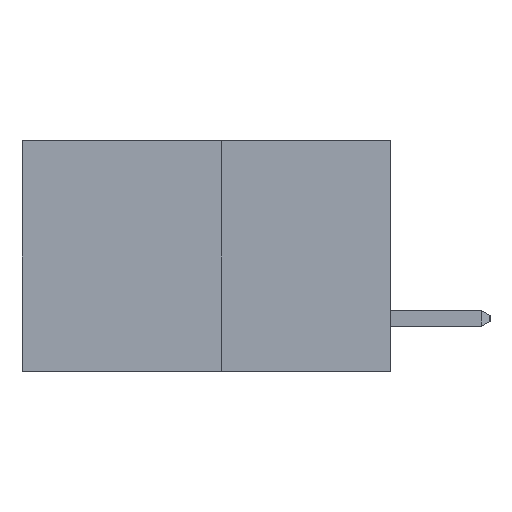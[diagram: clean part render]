
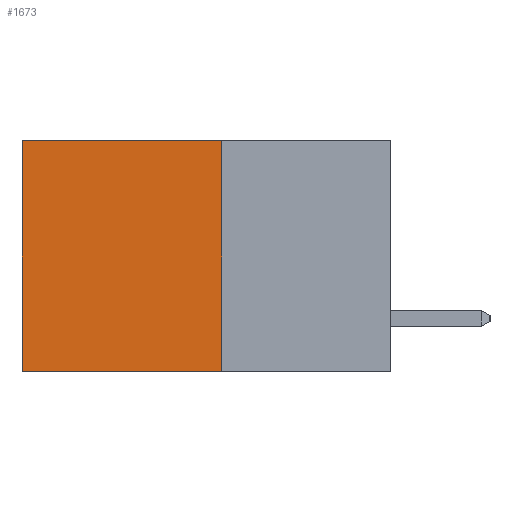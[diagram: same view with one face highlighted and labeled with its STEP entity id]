
A CAD part, left-side view. The second image highlights one B-rep face of the part: STEP entity #1673.
In plain terms, the highlighted planar face has unit normal (-1, 0, 0).
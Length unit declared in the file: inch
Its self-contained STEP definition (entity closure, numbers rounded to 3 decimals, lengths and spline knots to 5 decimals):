
#205 = LINE ( 'NONE', #525, #10479 ) ;
#525 = CARTESIAN_POINT ( 'NONE',  ( 0.277, 0.59, -0.37 ) ) ;
#1428 = VECTOR ( 'NONE', #2222, 39.37008 ) ;
#1673 = ADVANCED_FACE ( 'NONE', ( #11028 ), #9354, .F. ) ;
#1768 = VECTOR ( 'NONE', #6819, 39.37008 ) ;
#2113 = CARTESIAN_POINT ( 'NONE',  ( 0.277, 0.27, -0.37 ) ) ;
#2222 = DIRECTION ( 'NONE',  ( 0., 0., -1. ) ) ;
#2386 = LINE ( 'NONE', #12180, #1428 ) ;
#3002 = ORIENTED_EDGE ( 'NONE', *, *, #8285, .F. ) ;
#3289 = EDGE_CURVE ( 'NONE', #11826, #7920, #2386, .T. ) ;
#3498 = EDGE_CURVE ( 'NONE', #11826, #4639, #9947, .T. ) ;
#3953 = ORIENTED_EDGE ( 'NONE', *, *, #3498, .T. ) ;
#4101 = EDGE_LOOP ( 'NONE', ( #10529, #3002, #9128, #3953 ) ) ;
#4295 = AXIS2_PLACEMENT_3D ( 'NONE', #9626, #9228, #6537 ) ;
#4399 = CARTESIAN_POINT ( 'NONE',  ( 0.277, 0.27, -0.37 ) ) ;
#4639 = VERTEX_POINT ( 'NONE', #7911 ) ;
#5993 = VECTOR ( 'NONE', #12181, 39.37008 ) ;
#6537 = DIRECTION ( 'NONE',  ( 0., 0., -1. ) ) ;
#6768 = DIRECTION ( 'NONE',  ( 0., 0., -1. ) ) ;
#6819 = DIRECTION ( 'NONE',  ( 0., 1., 0. ) ) ;
#7879 = VERTEX_POINT ( 'NONE', #9518 ) ;
#7911 = CARTESIAN_POINT ( 'NONE',  ( 0.277, 0.59, 0. ) ) ;
#7920 = VERTEX_POINT ( 'NONE', #4399 ) ;
#8285 = EDGE_CURVE ( 'NONE', #7920, #7879, #8729, .T. ) ;
#8370 = CARTESIAN_POINT ( 'NONE',  ( 0.277, 0.27, 0. ) ) ;
#8729 = LINE ( 'NONE', #2113, #5993 ) ;
#9128 = ORIENTED_EDGE ( 'NONE', *, *, #3289, .F. ) ;
#9228 = DIRECTION ( 'NONE',  ( 1., 0., 0. ) ) ;
#9354 = PLANE ( 'NONE',  #4295 ) ;
#9518 = CARTESIAN_POINT ( 'NONE',  ( 0.277, 0.59, -0.37 ) ) ;
#9626 = CARTESIAN_POINT ( 'NONE',  ( 0.277, 0.27, -0.37 ) ) ;
#9632 = CARTESIAN_POINT ( 'NONE',  ( 0.277, 0.27, 0. ) ) ;
#9947 = LINE ( 'NONE', #8370, #1768 ) ;
#10479 = VECTOR ( 'NONE', #6768, 39.37008 ) ;
#10529 = ORIENTED_EDGE ( 'NONE', *, *, #12475, .T. ) ;
#11028 = FACE_OUTER_BOUND ( 'NONE', #4101, .T. ) ;
#11826 = VERTEX_POINT ( 'NONE', #9632 ) ;
#12180 = CARTESIAN_POINT ( 'NONE',  ( 0.277, 0.27, -0.37 ) ) ;
#12181 = DIRECTION ( 'NONE',  ( 0., 1., 0. ) ) ;
#12475 = EDGE_CURVE ( 'NONE', #4639, #7879, #205, .T. ) ;
